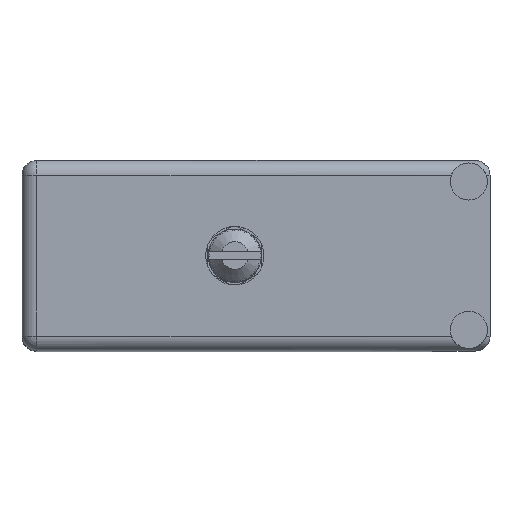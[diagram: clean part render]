
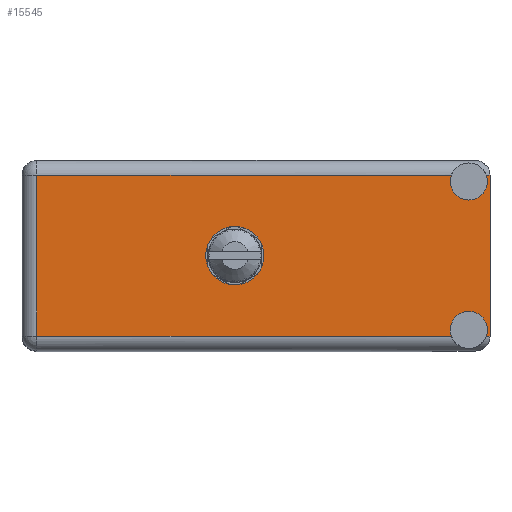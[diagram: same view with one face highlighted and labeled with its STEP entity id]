
A CAD part, top view. The second image highlights one B-rep face of the part: STEP entity #15545.
In plain terms, the highlighted face is planar.
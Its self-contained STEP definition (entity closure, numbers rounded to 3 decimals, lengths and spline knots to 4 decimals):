
#797 = CARTESIAN_POINT ( 'NONE',  ( 2.108, 1.566, -0.187 ) ) ;
#1520 = DIRECTION ( 'NONE',  ( -1., 0., 0. ) ) ;
#6456 = VECTOR ( 'NONE', #73284, 39.3701 ) ;
#6569 = DIRECTION ( 'NONE',  ( 0., 0., 1. ) ) ;
#7413 = DIRECTION ( 'NONE',  ( 0., 0., 1. ) ) ;
#7972 = DIRECTION ( 'NONE',  ( 0., 1., 0. ) ) ;
#8510 = EDGE_CURVE ( 'NONE', #33433, #28669, #55581, .T. ) ;
#9729 = AXIS2_PLACEMENT_3D ( 'NONE', #90999, #90426, #72686 ) ;
#10312 = CIRCLE ( 'NONE', #66889, 0.1375 ) ;
#10447 = VECTOR ( 'NONE', #79286, 39.3701 ) ;
#10737 = ORIENTED_EDGE ( 'NONE', *, *, #52585, .F. ) ;
#11204 = VERTEX_POINT ( 'NONE', #30773 ) ;
#11364 = CARTESIAN_POINT ( 'NONE',  ( 0.07, 1.566, -0.829 ) ) ;
#12206 = ORIENTED_EDGE ( 'NONE', *, *, #89871, .T. ) ;
#15545 = ADVANCED_FACE ( 'NONE', ( #34124, #103815 ), #78678, .T. ) ;
#17154 = AXIS2_PLACEMENT_3D ( 'NONE', #94800, #7972, #7413 ) ;
#18894 = CARTESIAN_POINT ( 'NONE',  ( 0., 1.566, -0.829 ) ) ;
#20007 = CARTESIAN_POINT ( 'NONE',  ( 2.108, 1.566, -0.0995 ) ) ;
#20429 = CARTESIAN_POINT ( 'NONE',  ( 2.208, 1.566, -0.07 ) ) ;
#20933 = ORIENTED_EDGE ( 'NONE', *, *, #55580, .F. ) ;
#21270 = DIRECTION ( 'NONE',  ( 0., 0., 1. ) ) ;
#24672 = EDGE_CURVE ( 'NONE', #32030, #33896, #69748, .T. ) ;
#24751 = EDGE_CURVE ( 'NONE', #25778, #97506, #86875, .T. ) ;
#25778 = VERTEX_POINT ( 'NONE', #797 ) ;
#26469 = CARTESIAN_POINT ( 'NONE',  ( 2.0256, 1.566, -0.829 ) ) ;
#26677 = DIRECTION ( 'NONE',  ( 0., 1., 0. ) ) ;
#27360 = EDGE_CURVE ( 'NONE', #100875, #97506, #62157, .T. ) ;
#28669 = VERTEX_POINT ( 'NONE', #56278 ) ;
#29162 = DIRECTION ( 'NONE',  ( 0., 0., 1. ) ) ;
#29768 = ORIENTED_EDGE ( 'NONE', *, *, #27360, .T. ) ;
#29854 = CARTESIAN_POINT ( 'NONE',  ( 0.07, 1.566, -0.899 ) ) ;
#30773 = CARTESIAN_POINT ( 'NONE',  ( 1.004, 1.566, -0.312 ) ) ;
#32030 = VERTEX_POINT ( 'NONE', #26469 ) ;
#33433 = VERTEX_POINT ( 'NONE', #50021 ) ;
#33896 = VERTEX_POINT ( 'NONE', #11364 ) ;
#34124 = FACE_BOUND ( 'NONE', #101856, .T. ) ;
#40136 = ORIENTED_EDGE ( 'NONE', *, *, #24751, .F. ) ;
#43480 = VECTOR ( 'NONE', #60849, 39.3701 ) ;
#44037 = ORIENTED_EDGE ( 'NONE', *, *, #101888, .T. ) ;
#44086 = DIRECTION ( 'NONE',  ( -1., 0., 0. ) ) ;
#44422 = CIRCLE ( 'NONE', #9729, 0.0875 ) ;
#44963 = LINE ( 'NONE', #79758, #61055 ) ;
#46024 = DIRECTION ( 'NONE',  ( 0., 1., 0. ) ) ;
#46725 = CARTESIAN_POINT ( 'NONE',  ( 2.1904, 1.566, -0.829 ) ) ;
#46767 = AXIS2_PLACEMENT_3D ( 'NONE', #108783, #46024, #80265 ) ;
#46879 = CARTESIAN_POINT ( 'NONE',  ( 1.004, 1.566, -0.587 ) ) ;
#50021 = CARTESIAN_POINT ( 'NONE',  ( 2.1904, 1.566, -0.07 ) ) ;
#51202 = CARTESIAN_POINT ( 'NONE',  ( 1.004, 1.566, -0.4495 ) ) ;
#51746 = VERTEX_POINT ( 'NONE', #46725 ) ;
#52227 = AXIS2_PLACEMENT_3D ( 'NONE', #20007, #90855, #29162 ) ;
#52585 = EDGE_CURVE ( 'NONE', #32030, #72178, #44422, .T. ) ;
#53272 = VERTEX_POINT ( 'NONE', #86221 ) ;
#55580 = EDGE_CURVE ( 'NONE', #33433, #25778, #92016, .T. ) ;
#55581 = LINE ( 'NONE', #81860, #6456 ) ;
#56278 = CARTESIAN_POINT ( 'NONE',  ( 2.208, 1.566, -0.07 ) ) ;
#60849 = DIRECTION ( 'NONE',  ( 0., 0., 1. ) ) ;
#60890 = EDGE_CURVE ( 'NONE', #11204, #76036, #96013, .T. ) ;
#61055 = VECTOR ( 'NONE', #1520, 39.3701 ) ;
#62157 = LINE ( 'NONE', #20429, #10447 ) ;
#64078 = CARTESIAN_POINT ( 'NONE',  ( 2.0256, 1.566, -0.07 ) ) ;
#66788 = VECTOR ( 'NONE', #44086, 39.3701 ) ;
#66889 = AXIS2_PLACEMENT_3D ( 'NONE', #51202, #78575, #68299 ) ;
#67278 = AXIS2_PLACEMENT_3D ( 'NONE', #77355, #84823, #6569 ) ;
#68299 = DIRECTION ( 'NONE',  ( 0., 0., 1. ) ) ;
#69748 = LINE ( 'NONE', #18894, #66788 ) ;
#70086 = CARTESIAN_POINT ( 'NONE',  ( 0., 1.566, -0.899 ) ) ;
#72178 = VERTEX_POINT ( 'NONE', #72580 ) ;
#72580 = CARTESIAN_POINT ( 'NONE',  ( 2.108, 1.566, -0.712 ) ) ;
#72686 = DIRECTION ( 'NONE',  ( 0., 0., 1. ) ) ;
#73284 = DIRECTION ( 'NONE',  ( 1., 0., 0. ) ) ;
#74879 = ORIENTED_EDGE ( 'NONE', *, *, #60890, .F. ) ;
#76036 = VERTEX_POINT ( 'NONE', #46879 ) ;
#76841 = CARTESIAN_POINT ( 'NONE',  ( 2.208, 1.566, 0. ) ) ;
#77355 = CARTESIAN_POINT ( 'NONE',  ( 2.108, 1.566, -0.7995 ) ) ;
#78575 = DIRECTION ( 'NONE',  ( 0., 1., 0. ) ) ;
#78678 = PLANE ( 'NONE',  #96937 ) ;
#79286 = DIRECTION ( 'NONE',  ( 1., 0., 0. ) ) ;
#79758 = CARTESIAN_POINT ( 'NONE',  ( 0., 1.566, -0.829 ) ) ;
#80265 = DIRECTION ( 'NONE',  ( 0., 0., 1. ) ) ;
#81860 = CARTESIAN_POINT ( 'NONE',  ( 2.208, 1.566, -0.07 ) ) ;
#84823 = DIRECTION ( 'NONE',  ( 0., 1., 0. ) ) ;
#85337 = VECTOR ( 'NONE', #21270, 39.3701 ) ;
#86221 = CARTESIAN_POINT ( 'NONE',  ( 2.208, 1.566, -0.829 ) ) ;
#86348 = ORIENTED_EDGE ( 'NONE', *, *, #95953, .F. ) ;
#86875 = CIRCLE ( 'NONE', #52227, 0.0875 ) ;
#89871 = EDGE_CURVE ( 'NONE', #53272, #51746, #44963, .T. ) ;
#90426 = DIRECTION ( 'NONE',  ( 0., 1., 0. ) ) ;
#90855 = DIRECTION ( 'NONE',  ( 0., 1., 0. ) ) ;
#90999 = CARTESIAN_POINT ( 'NONE',  ( 2.108, 1.566, -0.7995 ) ) ;
#92016 = CIRCLE ( 'NONE', #17154, 0.0875 ) ;
#93189 = ORIENTED_EDGE ( 'NONE', *, *, #8510, .T. ) ;
#93580 = EDGE_LOOP ( 'NONE', ( #29768, #40136, #20933, #93189, #112169, #12206, #101300, #10737, #100506, #44037 ) ) ;
#93583 = DIRECTION ( 'NONE',  ( 0., 0., 1. ) ) ;
#94800 = CARTESIAN_POINT ( 'NONE',  ( 2.108, 1.566, -0.0995 ) ) ;
#95953 = EDGE_CURVE ( 'NONE', #76036, #11204, #10312, .T. ) ;
#96013 = CIRCLE ( 'NONE', #46767, 0.1375 ) ;
#96937 = AXIS2_PLACEMENT_3D ( 'NONE', #70086, #26677, #93583 ) ;
#97506 = VERTEX_POINT ( 'NONE', #64078 ) ;
#100506 = ORIENTED_EDGE ( 'NONE', *, *, #24672, .T. ) ;
#100875 = VERTEX_POINT ( 'NONE', #103434 ) ;
#101300 = ORIENTED_EDGE ( 'NONE', *, *, #103836, .F. ) ;
#101856 = EDGE_LOOP ( 'NONE', ( #74879, #86348 ) ) ;
#101888 = EDGE_CURVE ( 'NONE', #33896, #100875, #106946, .T. ) ;
#103434 = CARTESIAN_POINT ( 'NONE',  ( 0.07, 1.566, -0.07 ) ) ;
#103815 = FACE_OUTER_BOUND ( 'NONE', #93580, .T. ) ;
#103836 = EDGE_CURVE ( 'NONE', #72178, #51746, #112861, .T. ) ;
#106946 = LINE ( 'NONE', #29854, #85337 ) ;
#108783 = CARTESIAN_POINT ( 'NONE',  ( 1.004, 1.566, -0.4495 ) ) ;
#111127 = LINE ( 'NONE', #76841, #43480 ) ;
#111538 = EDGE_CURVE ( 'NONE', #53272, #28669, #111127, .T. ) ;
#112169 = ORIENTED_EDGE ( 'NONE', *, *, #111538, .F. ) ;
#112861 = CIRCLE ( 'NONE', #67278, 0.0875 ) ;
